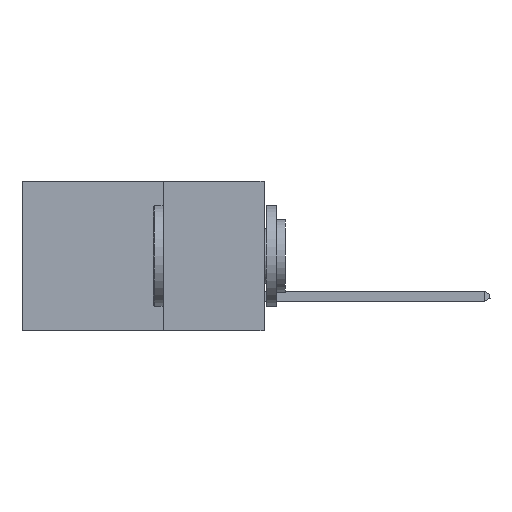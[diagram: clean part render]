
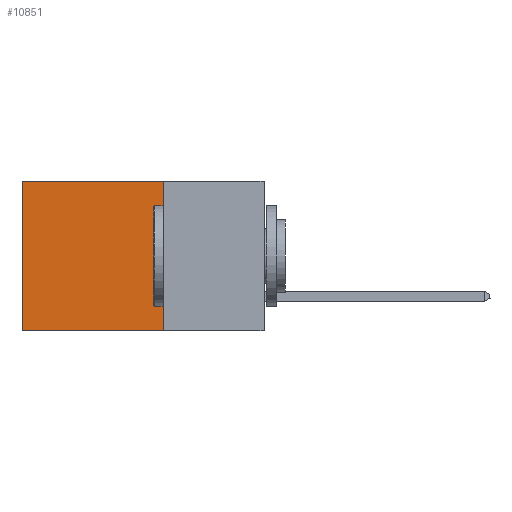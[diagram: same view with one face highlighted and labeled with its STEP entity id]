
A CAD part, left-side view. The second image highlights one B-rep face of the part: STEP entity #10851.
In plain terms, the highlighted planar face has unit normal (-1, 0, 0).
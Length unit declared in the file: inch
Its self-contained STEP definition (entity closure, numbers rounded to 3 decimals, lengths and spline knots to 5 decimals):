
#545 = EDGE_CURVE ( 'NONE', #13463, #19430, #7483, .T. ) ;
#758 = CARTESIAN_POINT ( 'NONE',  ( 0.298, 0.25, 0. ) ) ;
#1201 = CARTESIAN_POINT ( 'NONE',  ( 0.298, 0.6, -0.37 ) ) ;
#1341 = EDGE_CURVE ( 'NONE', #9103, #13463, #13453, .T. ) ;
#2193 = ORIENTED_EDGE ( 'NONE', *, *, #16395, .F. ) ;
#2314 = DIRECTION ( 'NONE',  ( 0., 0., -1. ) ) ;
#4597 = LINE ( 'NONE', #7052, #5393 ) ;
#5012 = DIRECTION ( 'NONE',  ( 1., 0., 0. ) ) ;
#5393 = VECTOR ( 'NONE', #14032, 39.37008 ) ;
#5993 = DIRECTION ( 'NONE',  ( 0., 1., 0. ) ) ;
#6130 = VECTOR ( 'NONE', #22052, 39.37008 ) ;
#6291 = CARTESIAN_POINT ( 'NONE',  ( 0.298, 0.6, 0. ) ) ;
#6721 = AXIS2_PLACEMENT_3D ( 'NONE', #22485, #5012, #17423 ) ;
#7052 = CARTESIAN_POINT ( 'NONE',  ( 0.298, 0.25, -0.37 ) ) ;
#7483 = LINE ( 'NONE', #19998, #6130 ) ;
#7852 = LINE ( 'NONE', #758, #11135 ) ;
#9103 = VERTEX_POINT ( 'NONE', #21985 ) ;
#10851 = ADVANCED_FACE ( 'NONE', ( #14279 ), #18962, .F. ) ;
#11135 = VECTOR ( 'NONE', #2314, 39.37008 ) ;
#12095 = VECTOR ( 'NONE', #5993, 39.37008 ) ;
#13453 = LINE ( 'NONE', #16475, #12095 ) ;
#13463 = VERTEX_POINT ( 'NONE', #6291 ) ;
#13666 = EDGE_CURVE ( 'NONE', #21688, #19430, #4597, .T. ) ;
#13848 = CARTESIAN_POINT ( 'NONE',  ( 0.298, 0.25, -0.37 ) ) ;
#14032 = DIRECTION ( 'NONE',  ( 0., 1., 0. ) ) ;
#14098 = ORIENTED_EDGE ( 'NONE', *, *, #13666, .F. ) ;
#14279 = FACE_OUTER_BOUND ( 'NONE', #16682, .T. ) ;
#15665 = ORIENTED_EDGE ( 'NONE', *, *, #1341, .T. ) ;
#16395 = EDGE_CURVE ( 'NONE', #9103, #21688, #7852, .T. ) ;
#16475 = CARTESIAN_POINT ( 'NONE',  ( 0.298, 0.25, 0. ) ) ;
#16682 = EDGE_LOOP ( 'NONE', ( #18458, #14098, #2193, #15665 ) ) ;
#17423 = DIRECTION ( 'NONE',  ( 0., 0., -1. ) ) ;
#18458 = ORIENTED_EDGE ( 'NONE', *, *, #545, .T. ) ;
#18962 = PLANE ( 'NONE',  #6721 ) ;
#19430 = VERTEX_POINT ( 'NONE', #1201 ) ;
#19998 = CARTESIAN_POINT ( 'NONE',  ( 0.298, 0.6, 0. ) ) ;
#21688 = VERTEX_POINT ( 'NONE', #13848 ) ;
#21985 = CARTESIAN_POINT ( 'NONE',  ( 0.298, 0.25, 0. ) ) ;
#22052 = DIRECTION ( 'NONE',  ( 0., 0., -1. ) ) ;
#22485 = CARTESIAN_POINT ( 'NONE',  ( 0.298, 0.25, 0. ) ) ;
